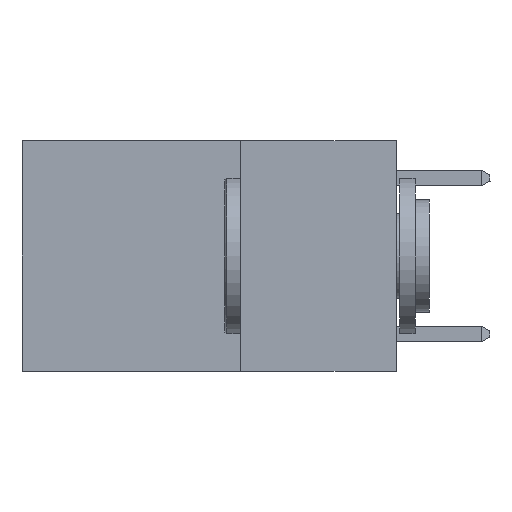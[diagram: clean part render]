
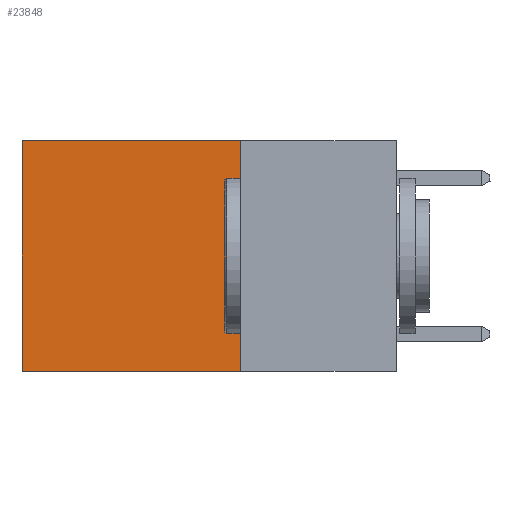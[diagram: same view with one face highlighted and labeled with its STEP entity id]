
A CAD part, left-side view. The second image highlights one B-rep face of the part: STEP entity #23848.
In plain terms, the highlighted planar face has unit normal (-1, 0, 0).
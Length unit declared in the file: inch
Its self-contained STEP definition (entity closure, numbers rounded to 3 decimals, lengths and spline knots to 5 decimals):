
#746 = LINE ( 'NONE', #16939, #17616 ) ;
#832 = LINE ( 'NONE', #4200, #24385 ) ;
#2072 = ORIENTED_EDGE ( 'NONE', *, *, #18670, .T. ) ;
#2690 = CARTESIAN_POINT ( 'NONE',  ( 0.2625, 0.25, 0. ) ) ;
#2832 = LINE ( 'NONE', #2690, #25598 ) ;
#3120 = CARTESIAN_POINT ( 'NONE',  ( 0.2625, 0.25, 0. ) ) ;
#4200 = CARTESIAN_POINT ( 'NONE',  ( 0.2625, 0.25, -0.37 ) ) ;
#4708 = EDGE_CURVE ( 'NONE', #8119, #28405, #832, .T. ) ;
#5258 = ORIENTED_EDGE ( 'NONE', *, *, #17887, .F. ) ;
#5406 = DIRECTION ( 'NONE',  ( 0., 0., -1. ) ) ;
#6899 = ORIENTED_EDGE ( 'NONE', *, *, #4708, .F. ) ;
#7371 = ORIENTED_EDGE ( 'NONE', *, *, #11862, .T. ) ;
#8119 = VERTEX_POINT ( 'NONE', #27246 ) ;
#11862 = EDGE_CURVE ( 'NONE', #14093, #28405, #16964, .T. ) ;
#14093 = VERTEX_POINT ( 'NONE', #22903 ) ;
#14362 = AXIS2_PLACEMENT_3D ( 'NONE', #3120, #19173, #5406 ) ;
#14733 = DIRECTION ( 'NONE',  ( 0., 0., -1. ) ) ;
#15498 = VECTOR ( 'NONE', #27737, 39.37008 ) ;
#16471 = DIRECTION ( 'NONE',  ( 0., 1., 0. ) ) ;
#16753 = CARTESIAN_POINT ( 'NONE',  ( 0.2625, 0.6, -0.37 ) ) ;
#16906 = PLANE ( 'NONE',  #14362 ) ;
#16939 = CARTESIAN_POINT ( 'NONE',  ( 0.2625, 0.25, 0. ) ) ;
#16964 = LINE ( 'NONE', #25580, #15498 ) ;
#17616 = VECTOR ( 'NONE', #14733, 39.37008 ) ;
#17887 = EDGE_CURVE ( 'NONE', #28610, #8119, #746, .T. ) ;
#18670 = EDGE_CURVE ( 'NONE', #28610, #14093, #2832, .T. ) ;
#19173 = DIRECTION ( 'NONE',  ( 1., 0., 0. ) ) ;
#22903 = CARTESIAN_POINT ( 'NONE',  ( 0.2625, 0.6, 0. ) ) ;
#23290 = EDGE_LOOP ( 'NONE', ( #7371, #6899, #5258, #2072 ) ) ;
#23848 = ADVANCED_FACE ( 'NONE', ( #25343 ), #16906, .F. ) ;
#24385 = VECTOR ( 'NONE', #26911, 39.37008 ) ;
#25343 = FACE_OUTER_BOUND ( 'NONE', #23290, .T. ) ;
#25580 = CARTESIAN_POINT ( 'NONE',  ( 0.2625, 0.6, 0. ) ) ;
#25598 = VECTOR ( 'NONE', #16471, 39.37008 ) ;
#26911 = DIRECTION ( 'NONE',  ( 0., 1., 0. ) ) ;
#27246 = CARTESIAN_POINT ( 'NONE',  ( 0.2625, 0.25, -0.37 ) ) ;
#27737 = DIRECTION ( 'NONE',  ( 0., 0., -1. ) ) ;
#28405 = VERTEX_POINT ( 'NONE', #16753 ) ;
#28485 = CARTESIAN_POINT ( 'NONE',  ( 0.2625, 0.25, 0. ) ) ;
#28610 = VERTEX_POINT ( 'NONE', #28485 ) ;
